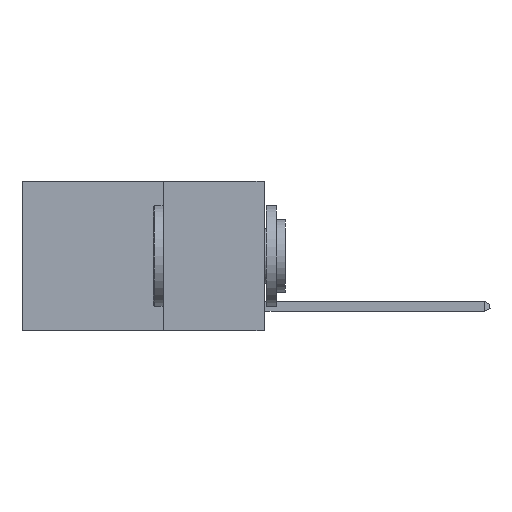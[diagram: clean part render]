
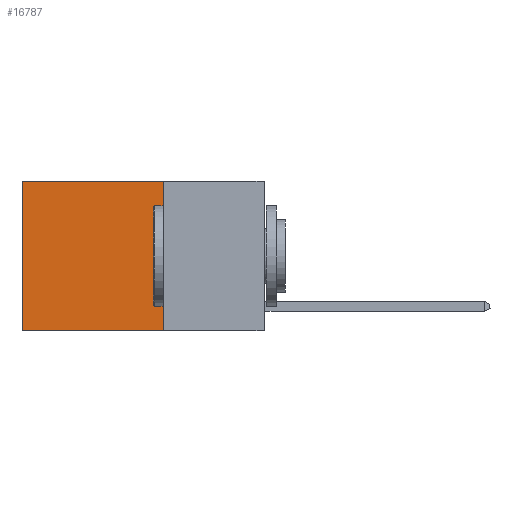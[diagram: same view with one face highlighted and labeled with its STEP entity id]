
A CAD part, left-side view. The second image highlights one B-rep face of the part: STEP entity #16787.
In plain terms, the highlighted planar face has unit normal (-1, 0, 0).
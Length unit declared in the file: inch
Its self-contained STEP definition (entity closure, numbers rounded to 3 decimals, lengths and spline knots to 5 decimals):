
#456 = VECTOR ( 'NONE', #3579, 39.37008 ) ;
#743 = CARTESIAN_POINT ( 'NONE',  ( 0.2625, 0.25, 0. ) ) ;
#1256 = EDGE_CURVE ( 'NONE', #11886, #1850, #3665, .T. ) ;
#1525 = CARTESIAN_POINT ( 'NONE',  ( 0.2625, 0.6, -0.37 ) ) ;
#1850 = VERTEX_POINT ( 'NONE', #8435 ) ;
#2371 = CARTESIAN_POINT ( 'NONE',  ( 0.2625, 0.25, 0. ) ) ;
#2621 = EDGE_CURVE ( 'NONE', #5029, #4931, #3687, .T. ) ;
#2903 = EDGE_CURVE ( 'NONE', #1850, #4931, #16562, .T. ) ;
#3329 = DIRECTION ( 'NONE',  ( 0., 1., 0. ) ) ;
#3579 = DIRECTION ( 'NONE',  ( 0., 0., -1. ) ) ;
#3665 = LINE ( 'NONE', #2371, #4344 ) ;
#3687 = LINE ( 'NONE', #15519, #10244 ) ;
#4344 = VECTOR ( 'NONE', #3329, 39.37008 ) ;
#4931 = VERTEX_POINT ( 'NONE', #1525 ) ;
#4946 = LINE ( 'NONE', #10153, #6944 ) ;
#5029 = VERTEX_POINT ( 'NONE', #7435 ) ;
#5239 = DIRECTION ( 'NONE',  ( 0., 1., 0. ) ) ;
#5534 = PLANE ( 'NONE',  #12600 ) ;
#6674 = FACE_OUTER_BOUND ( 'NONE', #15214, .T. ) ;
#6944 = VECTOR ( 'NONE', #15414, 39.37008 ) ;
#7435 = CARTESIAN_POINT ( 'NONE',  ( 0.2625, 0.25, -0.37 ) ) ;
#7534 = ORIENTED_EDGE ( 'NONE', *, *, #2903, .T. ) ;
#8197 = DIRECTION ( 'NONE',  ( 0., 0., -1. ) ) ;
#8435 = CARTESIAN_POINT ( 'NONE',  ( 0.2625, 0.6, 0. ) ) ;
#8682 = ORIENTED_EDGE ( 'NONE', *, *, #2621, .F. ) ;
#9762 = EDGE_CURVE ( 'NONE', #11886, #5029, #4946, .T. ) ;
#9993 = CARTESIAN_POINT ( 'NONE',  ( 0.2625, 0.6, 0. ) ) ;
#10153 = CARTESIAN_POINT ( 'NONE',  ( 0.2625, 0.25, 0. ) ) ;
#10244 = VECTOR ( 'NONE', #5239, 39.37008 ) ;
#10560 = CARTESIAN_POINT ( 'NONE',  ( 0.2625, 0.25, 0. ) ) ;
#11633 = ORIENTED_EDGE ( 'NONE', *, *, #1256, .T. ) ;
#11886 = VERTEX_POINT ( 'NONE', #743 ) ;
#12031 = DIRECTION ( 'NONE',  ( 1., 0., 0. ) ) ;
#12600 = AXIS2_PLACEMENT_3D ( 'NONE', #10560, #12031, #8197 ) ;
#15214 = EDGE_LOOP ( 'NONE', ( #7534, #8682, #15296, #11633 ) ) ;
#15296 = ORIENTED_EDGE ( 'NONE', *, *, #9762, .F. ) ;
#15414 = DIRECTION ( 'NONE',  ( 0., 0., -1. ) ) ;
#15519 = CARTESIAN_POINT ( 'NONE',  ( 0.2625, 0.25, -0.37 ) ) ;
#16562 = LINE ( 'NONE', #9993, #456 ) ;
#16787 = ADVANCED_FACE ( 'NONE', ( #6674 ), #5534, .F. ) ;
